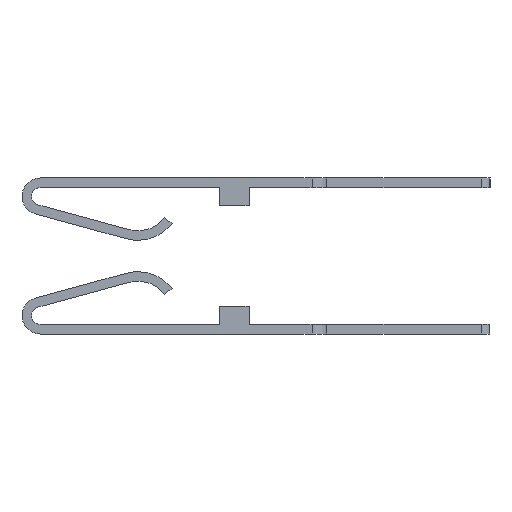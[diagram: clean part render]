
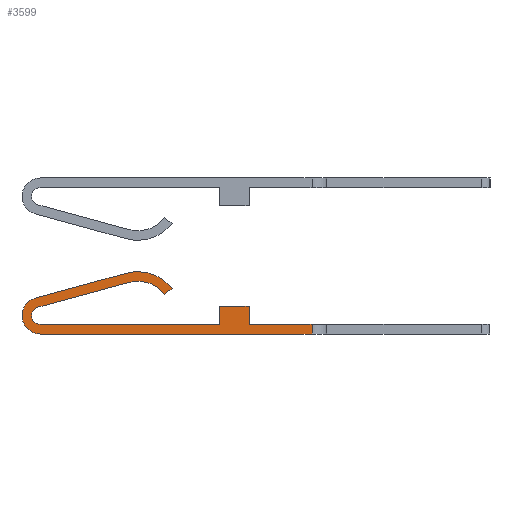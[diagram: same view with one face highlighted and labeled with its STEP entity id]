
A CAD part, left-side view. The second image highlights one B-rep face of the part: STEP entity #3599.
In plain terms, the highlighted face is planar.
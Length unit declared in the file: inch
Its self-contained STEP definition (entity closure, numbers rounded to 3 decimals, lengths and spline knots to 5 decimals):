
#31 = VECTOR ( 'NONE', #17769, 39.37008 ) ;
#88 = CARTESIAN_POINT ( 'NONE',  ( 0.05422, 0.11518, 0.0445 ) ) ;
#180 = CARTESIAN_POINT ( 'NONE',  ( 0., 0.285, 0.0445 ) ) ;
#186 = VERTEX_POINT ( 'NONE', #2135 ) ;
#270 = VECTOR ( 'NONE', #18686, 39.37008 ) ;
#545 = CARTESIAN_POINT ( 'NONE',  ( 0.025, 0.285, 0.0445 ) ) ;
#675 = EDGE_CURVE ( 'NONE', #7022, #11021, #19495, .T. ) ;
#721 = DIRECTION ( 'NONE',  ( -1., 0., 0. ) ) ;
#785 = FACE_OUTER_BOUND ( 'NONE', #15097, .T. ) ;
#873 = LINE ( 'NONE', #958, #9332 ) ;
#958 = CARTESIAN_POINT ( 'NONE',  ( 0.038, 0., 0.0445 ) ) ;
#974 = VERTEX_POINT ( 'NONE', #17591 ) ;
#1246 = VECTOR ( 'NONE', #17672, 39.37008 ) ;
#1414 = DIRECTION ( 'NONE',  ( 0., -1., 0. ) ) ;
#1498 = DIRECTION ( 'NONE',  ( 1., 0., 0. ) ) ;
#1937 = LINE ( 'NONE', #3959, #5954 ) ;
#2135 = CARTESIAN_POINT ( 'NONE',  ( 0., -0.086, 0.0445 ) ) ;
#2230 = VECTOR ( 'NONE', #8672, 39.37008 ) ;
#2321 = EDGE_CURVE ( 'NONE', #17986, #7834, #1937, .T. ) ;
#2501 = CIRCLE ( 'NONE', #9644, 0.025 ) ;
#2623 = CARTESIAN_POINT ( 'NONE',  ( 0.03658, 0.28816, 0.0445 ) ) ;
#2743 = DIRECTION ( 'NONE',  ( 0., -1., 0. ) ) ;
#3599 = ADVANCED_FACE ( 'NONE', ( #785 ), #9143, .F. ) ;
#3839 = CARTESIAN_POINT ( 'NONE',  ( 0.04912, 0.29158, 0.0445 ) ) ;
#3959 = CARTESIAN_POINT ( 'NONE',  ( 0.0623, 0.105, 0.0445 ) ) ;
#4090 = CARTESIAN_POINT ( 'NONE',  ( 0.013, 0.04, 0.0445 ) ) ;
#4853 = CARTESIAN_POINT ( 'NONE',  ( 0., 0., 0.0445 ) ) ;
#4979 = CARTESIAN_POINT ( 'NONE',  ( 0.038, 0.04, 0.0445 ) ) ;
#5070 = DIRECTION ( 'NONE',  ( 0., 0., 1. ) ) ;
#5443 = ORIENTED_EDGE ( 'NONE', *, *, #13499, .T. ) ;
#5476 = LINE ( 'NONE', #2623, #270 ) ;
#5691 = EDGE_CURVE ( 'NONE', #18294, #974, #18048, .T. ) ;
#5881 = EDGE_CURVE ( 'NONE', #8069, #20570, #18740, .T. ) ;
#5954 = VECTOR ( 'NONE', #14995, 39.37008 ) ;
#6374 = ORIENTED_EDGE ( 'NONE', *, *, #8054, .T. ) ;
#7022 = VERTEX_POINT ( 'NONE', #15180 ) ;
#7210 = AXIS2_PLACEMENT_3D ( 'NONE', #9075, #10785, #721 ) ;
#7320 = CARTESIAN_POINT ( 'NONE',  ( 0.025, 0.152, 0.0445 ) ) ;
#7483 = LINE ( 'NONE', #17647, #15066 ) ;
#7619 = ORIENTED_EDGE ( 'NONE', *, *, #13269, .F. ) ;
#7755 = ORIENTED_EDGE ( 'NONE', *, *, #5691, .T. ) ;
#7834 = VERTEX_POINT ( 'NONE', #11053 ) ;
#7856 = ORIENTED_EDGE ( 'NONE', *, *, #12411, .F. ) ;
#8054 = EDGE_CURVE ( 'NONE', #186, #10782, #18813, .T. ) ;
#8069 = VERTEX_POINT ( 'NONE', #4979 ) ;
#8188 = CARTESIAN_POINT ( 'NONE',  ( 0.013, -0.086, 0.0445 ) ) ;
#8406 = ORIENTED_EDGE ( 'NONE', *, *, #5881, .T. ) ;
#8561 = ORIENTED_EDGE ( 'NONE', *, *, #17814, .T. ) ;
#8672 = DIRECTION ( 'NONE',  ( 0., -1., 0. ) ) ;
#8914 = VERTEX_POINT ( 'NONE', #180 ) ;
#8977 = DIRECTION ( 'NONE',  ( -1., 0., 0. ) ) ;
#9075 = CARTESIAN_POINT ( 'NONE',  ( 0.025, 0.285, 0.0445 ) ) ;
#9143 = PLANE ( 'NONE',  #7210 ) ;
#9156 = CIRCLE ( 'NONE', #11669, 0.047 ) ;
#9166 = ORIENTED_EDGE ( 'NONE', *, *, #675, .T. ) ;
#9190 = ORIENTED_EDGE ( 'NONE', *, *, #19552, .T. ) ;
#9332 = VECTOR ( 'NONE', #2743, 39.37008 ) ;
#9446 = EDGE_CURVE ( 'NONE', #17223, #19411, #20414, .T. ) ;
#9643 = ORIENTED_EDGE ( 'NONE', *, *, #10153, .T. ) ;
#9644 = AXIS2_PLACEMENT_3D ( 'NONE', #14784, #5070, #16338 ) ;
#9648 = CARTESIAN_POINT ( 'NONE',  ( 0.025, 0.152, 0.0445 ) ) ;
#9911 = VECTOR ( 'NONE', #15110, 39.37008 ) ;
#10153 = EDGE_CURVE ( 'NONE', #17442, #17986, #9156, .T. ) ;
#10280 = CARTESIAN_POINT ( 'NONE',  ( 0., 0., 0.0445 ) ) ;
#10489 = VECTOR ( 'NONE', #1498, 39.37008 ) ;
#10782 = VERTEX_POINT ( 'NONE', #8188 ) ;
#10785 = DIRECTION ( 'NONE',  ( 0., 0., -1. ) ) ;
#10884 = ORIENTED_EDGE ( 'NONE', *, *, #2321, .T. ) ;
#10939 = CARTESIAN_POINT ( 'NONE',  ( 0.013, 0., 0.0445 ) ) ;
#11021 = VERTEX_POINT ( 'NONE', #13506 ) ;
#11053 = CARTESIAN_POINT ( 'NONE',  ( 0.0623, 0.105, 0.0445 ) ) ;
#11263 = DIRECTION ( 'NONE',  ( -1., 0., 0. ) ) ;
#11423 = ORIENTED_EDGE ( 'NONE', *, *, #15861, .T. ) ;
#11468 = CIRCLE ( 'NONE', #20404, 0.06 ) ;
#11669 = AXIS2_PLACEMENT_3D ( 'NONE', #9648, #20539, #11263 ) ;
#11779 = ORIENTED_EDGE ( 'NONE', *, *, #9446, .T. ) ;
#11801 = ORIENTED_EDGE ( 'NONE', *, *, #20282, .T. ) ;
#12154 = CARTESIAN_POINT ( 'NONE',  ( 0.07034, 0.16437, 0.0445 ) ) ;
#12240 = DIRECTION ( 'NONE',  ( -1., 0., 0. ) ) ;
#12411 = EDGE_CURVE ( 'NONE', #8069, #974, #873, .T. ) ;
#13269 = EDGE_CURVE ( 'NONE', #18294, #10782, #7483, .T. ) ;
#13404 = LINE ( 'NONE', #16221, #31 ) ;
#13499 = EDGE_CURVE ( 'NONE', #8914, #186, #19355, .T. ) ;
#13506 = CARTESIAN_POINT ( 'NONE',  ( 0.03658, 0.28816, 0.0445 ) ) ;
#13529 = CARTESIAN_POINT ( 'NONE',  ( 0.038, 0.04, 0.0445 ) ) ;
#14784 = CARTESIAN_POINT ( 'NONE',  ( 0.025, 0.285, 0.0445 ) ) ;
#14995 = DIRECTION ( 'NONE',  ( 0.622, -0.783, 0. ) ) ;
#15066 = VECTOR ( 'NONE', #1414, 39.37008 ) ;
#15097 = EDGE_LOOP ( 'NONE', ( #5443, #6374, #7619, #7755, #7856, #8406, #8561, #9166, #9190, #9643, #10884, #11423, #11779, #11801 ) ) ;
#15110 = DIRECTION ( 'NONE',  ( -1., 0., 0. ) ) ;
#15180 = CARTESIAN_POINT ( 'NONE',  ( 0.013, 0.285, 0.0445 ) ) ;
#15861 = EDGE_CURVE ( 'NONE', #7834, #17223, #11468, .T. ) ;
#16221 = CARTESIAN_POINT ( 'NONE',  ( 0.013, 0., 0.0445 ) ) ;
#16338 = DIRECTION ( 'NONE',  ( -1., 0., 0. ) ) ;
#16416 = VECTOR ( 'NONE', #20689, 39.37008 ) ;
#17223 = VERTEX_POINT ( 'NONE', #19431 ) ;
#17442 = VERTEX_POINT ( 'NONE', #12154 ) ;
#17591 = CARTESIAN_POINT ( 'NONE',  ( 0.038, 0., 0.0445 ) ) ;
#17647 = CARTESIAN_POINT ( 'NONE',  ( 0.013, 0., 0.0445 ) ) ;
#17672 = DIRECTION ( 'NONE',  ( 1., 0., 0. ) ) ;
#17723 = CARTESIAN_POINT ( 'NONE',  ( -0.13841, -0.086, 0.0445 ) ) ;
#17769 = DIRECTION ( 'NONE',  ( 0., 1., 0. ) ) ;
#17814 = EDGE_CURVE ( 'NONE', #20570, #7022, #13404, .T. ) ;
#17986 = VERTEX_POINT ( 'NONE', #88 ) ;
#18048 = LINE ( 'NONE', #4853, #1246 ) ;
#18294 = VERTEX_POINT ( 'NONE', #10939 ) ;
#18438 = DIRECTION ( 'NONE',  ( 0., 0., 1. ) ) ;
#18686 = DIRECTION ( 'NONE',  ( 0.263, -0.965, 0. ) ) ;
#18740 = LINE ( 'NONE', #13529, #9911 ) ;
#18813 = LINE ( 'NONE', #17723, #10489 ) ;
#19207 = CARTESIAN_POINT ( 'NONE',  ( 0.04912, 0.29158, 0.0445 ) ) ;
#19355 = LINE ( 'NONE', #10280, #2230 ) ;
#19411 = VERTEX_POINT ( 'NONE', #3839 ) ;
#19431 = CARTESIAN_POINT ( 'NONE',  ( 0.08289, 0.16779, 0.0445 ) ) ;
#19495 = CIRCLE ( 'NONE', #19860, 0.012 ) ;
#19552 = EDGE_CURVE ( 'NONE', #11021, #17442, #5476, .T. ) ;
#19860 = AXIS2_PLACEMENT_3D ( 'NONE', #545, #19929, #12240 ) ;
#19929 = DIRECTION ( 'NONE',  ( 0., 0., -1. ) ) ;
#20282 = EDGE_CURVE ( 'NONE', #19411, #8914, #2501, .T. ) ;
#20404 = AXIS2_PLACEMENT_3D ( 'NONE', #7320, #18438, #8977 ) ;
#20414 = LINE ( 'NONE', #19207, #16416 ) ;
#20539 = DIRECTION ( 'NONE',  ( 0., 0., -1. ) ) ;
#20570 = VERTEX_POINT ( 'NONE', #4090 ) ;
#20689 = DIRECTION ( 'NONE',  ( -0.263, 0.965, 0. ) ) ;
